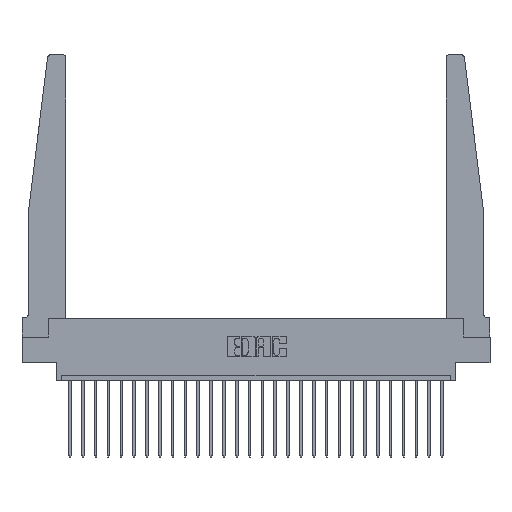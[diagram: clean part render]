
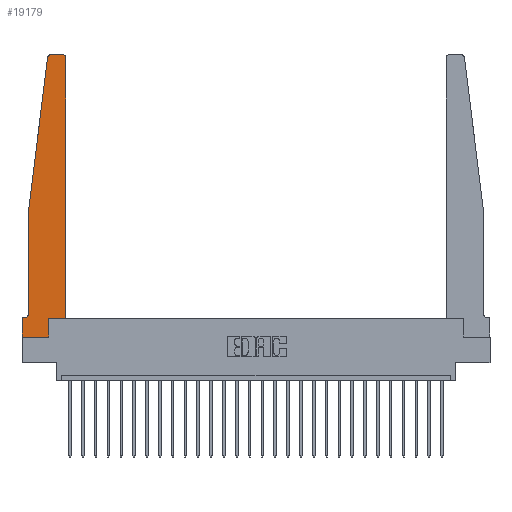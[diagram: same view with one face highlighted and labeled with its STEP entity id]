
A CAD part, top view. The second image highlights one B-rep face of the part: STEP entity #19179.
In plain terms, the highlighted planar face has unit normal (0, 0, 1).
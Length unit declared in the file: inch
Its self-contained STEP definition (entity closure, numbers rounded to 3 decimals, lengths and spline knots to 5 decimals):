
#61 = ORIENTED_EDGE ( 'NONE', *, *, #19090, .T. ) ;
#92 = DIRECTION ( 'NONE',  ( 1., 0., 0. ) ) ;
#281 = ORIENTED_EDGE ( 'NONE', *, *, #1493, .T. ) ;
#721 = VERTEX_POINT ( 'NONE', #15428 ) ;
#1122 = AXIS2_PLACEMENT_3D ( 'NONE', #4326, #17984, #6333 ) ;
#1171 = VECTOR ( 'NONE', #3478, 39.37008 ) ;
#1413 = DIRECTION ( 'NONE',  ( 1., 0., 0. ) ) ;
#1493 = EDGE_CURVE ( 'NONE', #4376, #8781, #2482, .T. ) ;
#1494 = EDGE_CURVE ( 'NONE', #23813, #8002, #13736, .T. ) ;
#1927 = EDGE_LOOP ( 'NONE', ( #18674, #10994, #14540, #7008, #281, #12457, #61, #7648, #13356, #8417, #13239, #20539 ) ) ;
#2175 = DIRECTION ( 'NONE',  ( 1., 0., 0. ) ) ;
#2482 = CIRCLE ( 'NONE', #21169, 0.05 ) ;
#2611 = CARTESIAN_POINT ( 'NONE',  ( 0.27653, 2.72, 0.37 ) ) ;
#2700 = VECTOR ( 'NONE', #22242, 39.37008 ) ;
#2762 = EDGE_CURVE ( 'NONE', #721, #16739, #11239, .T. ) ;
#2829 = EDGE_CURVE ( 'NONE', #8002, #8199, #20890, .T. ) ;
#3478 = DIRECTION ( 'NONE',  ( 0., 1., 0. ) ) ;
#3652 = CARTESIAN_POINT ( 'NONE',  ( 0.015, 0.2375, 0.37 ) ) ;
#3816 = AXIS2_PLACEMENT_3D ( 'NONE', #17376, #3956, #2175 ) ;
#3956 = DIRECTION ( 'NONE',  ( 0., 0., 1. ) ) ;
#4079 = CARTESIAN_POINT ( 'NONE',  ( 0.065, 0.1875, 0.37 ) ) ;
#4229 = CARTESIAN_POINT ( 'NONE',  ( 0.27653, 2.75, 0.37 ) ) ;
#4326 = CARTESIAN_POINT ( 'NONE',  ( 0., 0.1875, 0.37 ) ) ;
#4376 = VERTEX_POINT ( 'NONE', #5279 ) ;
#4964 = LINE ( 'NONE', #7921, #14686 ) ;
#5279 = CARTESIAN_POINT ( 'NONE',  ( 0.065, 0.2375, 0.37 ) ) ;
#5771 = DIRECTION ( 'NONE',  ( -1., 0., 0. ) ) ;
#5968 = DIRECTION ( 'NONE',  ( -0.122, -0.992, 0. ) ) ;
#6333 = DIRECTION ( 'NONE',  ( 1., 0., 0. ) ) ;
#6412 = CIRCLE ( 'NONE', #10319, 0.03 ) ;
#6450 = EDGE_CURVE ( 'NONE', #8199, #721, #22296, .T. ) ;
#6858 = CARTESIAN_POINT ( 'NONE',  ( 0.24675, 2.72367, 0.37 ) ) ;
#7008 = ORIENTED_EDGE ( 'NONE', *, *, #18869, .T. ) ;
#7018 = VECTOR ( 'NONE', #22434, 39.37008 ) ;
#7241 = VERTEX_POINT ( 'NONE', #20402 ) ;
#7648 = ORIENTED_EDGE ( 'NONE', *, *, #1494, .T. ) ;
#7893 = VERTEX_POINT ( 'NONE', #10043 ) ;
#7921 = CARTESIAN_POINT ( 'NONE',  ( 0.065, 1.25, 0.37 ) ) ;
#7962 = VERTEX_POINT ( 'NONE', #6858 ) ;
#8002 = VERTEX_POINT ( 'NONE', #24526 ) ;
#8199 = VERTEX_POINT ( 'NONE', #13109 ) ;
#8417 = ORIENTED_EDGE ( 'NONE', *, *, #6450, .T. ) ;
#8714 = CARTESIAN_POINT ( 'NONE',  ( 0.2605, 0.18, 0.37 ) ) ;
#8781 = VERTEX_POINT ( 'NONE', #15994 ) ;
#9573 = DIRECTION ( 'NONE',  ( 0., -1., 0. ) ) ;
#10043 = CARTESIAN_POINT ( 'NONE',  ( 0.065, 1.25, 0.37 ) ) ;
#10114 = PLANE ( 'NONE',  #1122 ) ;
#10188 = VECTOR ( 'NONE', #92, 39.37008 ) ;
#10319 = AXIS2_PLACEMENT_3D ( 'NONE', #2611, #21845, #18136 ) ;
#10994 = ORIENTED_EDGE ( 'NONE', *, *, #24465, .T. ) ;
#11065 = EDGE_CURVE ( 'NONE', #8781, #7241, #22049, .T. ) ;
#11239 = LINE ( 'NONE', #14685, #1171 ) ;
#11709 = DIRECTION ( 'NONE',  ( -1., 0., 0. ) ) ;
#11953 = LINE ( 'NONE', #15631, #24426 ) ;
#12188 = FACE_OUTER_BOUND ( 'NONE', #1927, .T. ) ;
#12457 = ORIENTED_EDGE ( 'NONE', *, *, #11065, .T. ) ;
#12875 = EDGE_CURVE ( 'NONE', #16739, #13504, #14063, .T. ) ;
#12880 = EDGE_CURVE ( 'NONE', #7962, #7893, #4964, .T. ) ;
#13109 = CARTESIAN_POINT ( 'NONE',  ( 0.2605, 0.18, 0.37 ) ) ;
#13239 = ORIENTED_EDGE ( 'NONE', *, *, #2762, .T. ) ;
#13356 = ORIENTED_EDGE ( 'NONE', *, *, #2829, .T. ) ;
#13504 = VERTEX_POINT ( 'NONE', #20694 ) ;
#13721 = CARTESIAN_POINT ( 'NONE',  ( 0.425, 0.18, 0.37 ) ) ;
#13736 = LINE ( 'NONE', #17307, #18275 ) ;
#14063 = CIRCLE ( 'NONE', #3816, 0.03 ) ;
#14528 = CARTESIAN_POINT ( 'NONE',  ( 0., 0., 0.37 ) ) ;
#14540 = ORIENTED_EDGE ( 'NONE', *, *, #12880, .T. ) ;
#14685 = CARTESIAN_POINT ( 'NONE',  ( 0.425, 0.18, 0.37 ) ) ;
#14686 = VECTOR ( 'NONE', #5968, 39.37008 ) ;
#15428 = CARTESIAN_POINT ( 'NONE',  ( 0.425, 0.18, 0.37 ) ) ;
#15631 = CARTESIAN_POINT ( 'NONE',  ( 0.25, 2.75, 0.37 ) ) ;
#15994 = CARTESIAN_POINT ( 'NONE',  ( 0.015, 0.1875, 0.37 ) ) ;
#16739 = VERTEX_POINT ( 'NONE', #21350 ) ;
#17069 = LINE ( 'NONE', #21744, #7018 ) ;
#17307 = CARTESIAN_POINT ( 'NONE',  ( 0., 0., 0.37 ) ) ;
#17376 = CARTESIAN_POINT ( 'NONE',  ( 0.395, 2.72, 0.37 ) ) ;
#17522 = CARTESIAN_POINT ( 'NONE',  ( 0.065, 1.25, 0.37 ) ) ;
#17681 = EDGE_CURVE ( 'NONE', #13504, #21082, #11953, .T. ) ;
#17984 = DIRECTION ( 'NONE',  ( 0., 0., 1. ) ) ;
#18136 = DIRECTION ( 'NONE',  ( 1., 0., 0. ) ) ;
#18262 = VECTOR ( 'NONE', #9573, 39.37008 ) ;
#18275 = VECTOR ( 'NONE', #1413, 39.37008 ) ;
#18674 = ORIENTED_EDGE ( 'NONE', *, *, #17681, .T. ) ;
#18869 = EDGE_CURVE ( 'NONE', #7893, #4376, #21890, .T. ) ;
#19090 = EDGE_CURVE ( 'NONE', #7241, #23813, #17069, .T. ) ;
#19179 = ADVANCED_FACE ( 'NONE', ( #12188 ), #10114, .T. ) ;
#20402 = CARTESIAN_POINT ( 'NONE',  ( 0., 0.1875, 0.37 ) ) ;
#20539 = ORIENTED_EDGE ( 'NONE', *, *, #12875, .T. ) ;
#20694 = CARTESIAN_POINT ( 'NONE',  ( 0.395, 2.75, 0.37 ) ) ;
#20890 = LINE ( 'NONE', #8714, #2700 ) ;
#20914 = DIRECTION ( 'NONE',  ( 0., 0., -1. ) ) ;
#21082 = VERTEX_POINT ( 'NONE', #4229 ) ;
#21169 = AXIS2_PLACEMENT_3D ( 'NONE', #3652, #20914, #24693 ) ;
#21350 = CARTESIAN_POINT ( 'NONE',  ( 0.425, 2.72, 0.37 ) ) ;
#21428 = VECTOR ( 'NONE', #5771, 39.37008 ) ;
#21744 = CARTESIAN_POINT ( 'NONE',  ( 0., 0., 0.37 ) ) ;
#21845 = DIRECTION ( 'NONE',  ( 0., 0., 1. ) ) ;
#21890 = LINE ( 'NONE', #17522, #18262 ) ;
#22049 = LINE ( 'NONE', #4079, #21428 ) ;
#22242 = DIRECTION ( 'NONE',  ( 0., 1., 0. ) ) ;
#22296 = LINE ( 'NONE', #13721, #10188 ) ;
#22434 = DIRECTION ( 'NONE',  ( 0., -1., 0. ) ) ;
#23813 = VERTEX_POINT ( 'NONE', #14528 ) ;
#24426 = VECTOR ( 'NONE', #11709, 39.37008 ) ;
#24465 = EDGE_CURVE ( 'NONE', #21082, #7962, #6412, .T. ) ;
#24526 = CARTESIAN_POINT ( 'NONE',  ( 0.2605, 0., 0.37 ) ) ;
#24693 = DIRECTION ( 'NONE',  ( -1., 0., 0. ) ) ;
